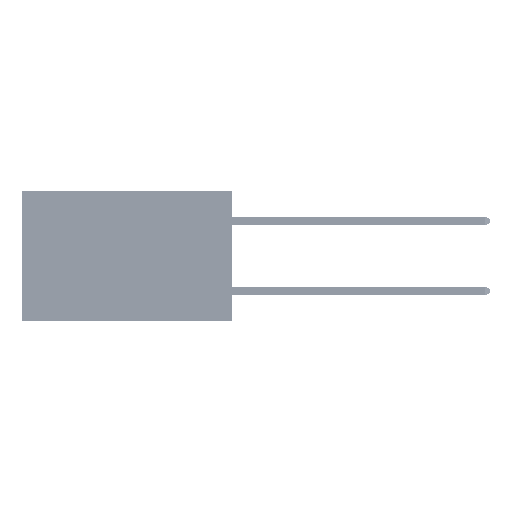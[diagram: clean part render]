
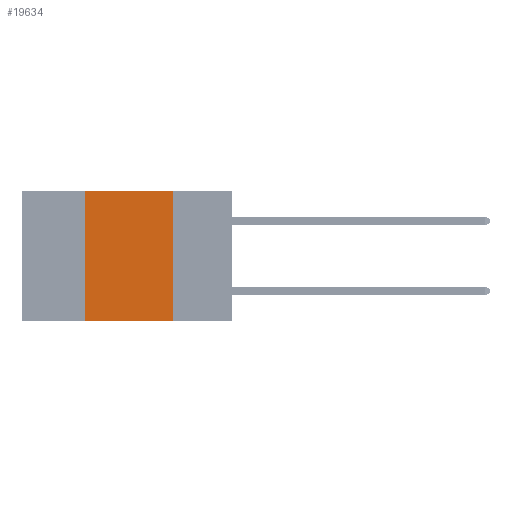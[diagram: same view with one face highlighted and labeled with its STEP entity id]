
A CAD part, left-side view. The second image highlights one B-rep face of the part: STEP entity #19634.
In plain terms, the highlighted planar face has unit normal (-1, 0, 0).
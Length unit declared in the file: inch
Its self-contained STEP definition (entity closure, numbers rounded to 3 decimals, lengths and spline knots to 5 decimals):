
#934 = VERTEX_POINT ( 'NONE', #49570 ) ;
#1229 = DIRECTION ( 'NONE',  ( 0., -1., 0. ) ) ;
#3286 = VECTOR ( 'NONE', #6045, 39.37008 ) ;
#4255 = DIRECTION ( 'NONE',  ( 1., 0., 0. ) ) ;
#5075 = LINE ( 'NONE', #20645, #20600 ) ;
#6045 = DIRECTION ( 'NONE',  ( 0., 0., -1. ) ) ;
#9326 = PLANE ( 'NONE',  #36996 ) ;
#9884 = LINE ( 'NONE', #25435, #3286 ) ;
#10851 = EDGE_LOOP ( 'NONE', ( #34618, #12732, #36835, #28402 ) ) ;
#12100 = CARTESIAN_POINT ( 'NONE',  ( 0., 0.42, -0.37 ) ) ;
#12732 = ORIENTED_EDGE ( 'NONE', *, *, #15581, .F. ) ;
#13740 = CARTESIAN_POINT ( 'NONE',  ( 0., 0.6, -0.37 ) ) ;
#15581 = EDGE_CURVE ( 'NONE', #19581, #42656, #5075, .T. ) ;
#16905 = EDGE_CURVE ( 'NONE', #29395, #934, #24462, .T. ) ;
#19189 = LINE ( 'NONE', #35025, #19487 ) ;
#19487 = VECTOR ( 'NONE', #23772, 39.37008 ) ;
#19581 = VERTEX_POINT ( 'NONE', #19822 ) ;
#19634 = ADVANCED_FACE ( 'NONE', ( #44323 ), #9326, .F. ) ;
#19822 = CARTESIAN_POINT ( 'NONE',  ( 0., 0.42, 0. ) ) ;
#20600 = VECTOR ( 'NONE', #36205, 39.37008 ) ;
#20645 = CARTESIAN_POINT ( 'NONE',  ( 0., 0.6, 0. ) ) ;
#23772 = DIRECTION ( 'NONE',  ( 0., 0., 1. ) ) ;
#24462 = LINE ( 'NONE', #13740, #49071 ) ;
#24881 = CARTESIAN_POINT ( 'NONE',  ( 0., 0.6, 0. ) ) ;
#25435 = CARTESIAN_POINT ( 'NONE',  ( 0., 0.17, 0. ) ) ;
#28402 = ORIENTED_EDGE ( 'NONE', *, *, #16905, .T. ) ;
#29395 = VERTEX_POINT ( 'NONE', #12100 ) ;
#31230 = EDGE_CURVE ( 'NONE', #29395, #19581, #19189, .T. ) ;
#34618 = ORIENTED_EDGE ( 'NONE', *, *, #46801, .F. ) ;
#35025 = CARTESIAN_POINT ( 'NONE',  ( 0., 0.42, 0. ) ) ;
#36205 = DIRECTION ( 'NONE',  ( 0., -1., 0. ) ) ;
#36835 = ORIENTED_EDGE ( 'NONE', *, *, #31230, .F. ) ;
#36996 = AXIS2_PLACEMENT_3D ( 'NONE', #24881, #4255, #47163 ) ;
#37199 = CARTESIAN_POINT ( 'NONE',  ( 0., 0.17, 0. ) ) ;
#42656 = VERTEX_POINT ( 'NONE', #37199 ) ;
#44323 = FACE_OUTER_BOUND ( 'NONE', #10851, .T. ) ;
#46801 = EDGE_CURVE ( 'NONE', #42656, #934, #9884, .T. ) ;
#47163 = DIRECTION ( 'NONE',  ( 0., 0., -1. ) ) ;
#49071 = VECTOR ( 'NONE', #1229, 39.37008 ) ;
#49570 = CARTESIAN_POINT ( 'NONE',  ( 0., 0.17, -0.37 ) ) ;
